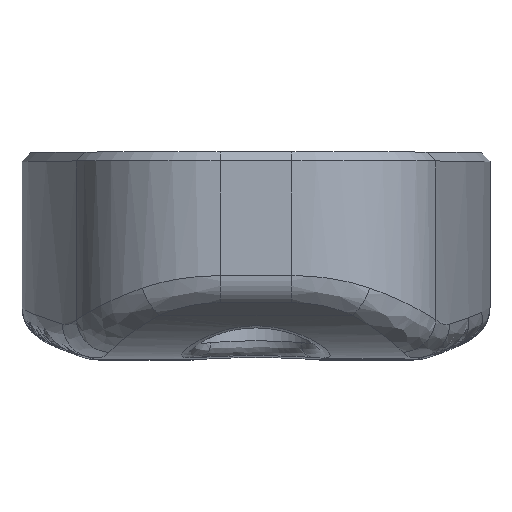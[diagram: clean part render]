
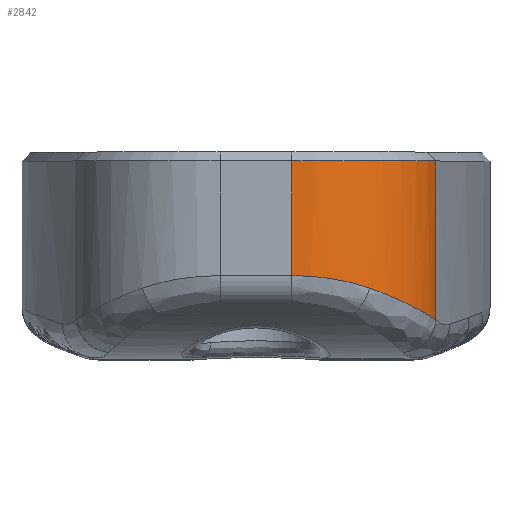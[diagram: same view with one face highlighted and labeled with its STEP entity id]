
A CAD part, top view. The second image highlights one B-rep face of the part: STEP entity #2842.
In plain terms, the highlighted cylindrical face has radius 10 mm (diameter 20 mm), a partial arc.
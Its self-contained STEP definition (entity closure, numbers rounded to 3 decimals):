
#208=LINE('',#6161,#362);
#209=LINE('',#6168,#363);
#362=VECTOR('',#3895,115.186);
#363=VECTOR('',#3898,10.);
#445=CYLINDRICAL_SURFACE('',#3165,10.);
#491=ELLIPSE('',#3166,11.484,10.);
#642=FACE_OUTER_BOUND('',#828,.T.);
#828=EDGE_LOOP('',(#2473,#2474,#2475,#2476,#2477));
#953=B_SPLINE_CURVE_WITH_KNOTS('',3,(#6171,#6172,#6173,#6174,#6175),
 .UNSPECIFIED.,.F.,.F.,(4,1,4),(0.,0.271,0.631),
 .UNSPECIFIED.);
#1103=CIRCLE('',#3154,10.);
#1340=VERTEX_POINT('',#6127);
#1342=VERTEX_POINT('',#6135);
#1347=VERTEX_POINT('',#6160);
#1348=VERTEX_POINT('',#6167);
#1349=VERTEX_POINT('',#6169);
#1726=EDGE_CURVE('',#1340,#1342,#1103,.T.);
#1738=EDGE_CURVE('',#1342,#1347,#208,.T.);
#1740=EDGE_CURVE('',#1340,#1348,#209,.T.);
#1741=EDGE_CURVE('',#1349,#1348,#491,.T.);
#1742=EDGE_CURVE('',#1347,#1349,#953,.T.);
#2473=ORIENTED_EDGE('',*,*,#1726,.F.);
#2474=ORIENTED_EDGE('',*,*,#1740,.T.);
#2475=ORIENTED_EDGE('',*,*,#1741,.F.);
#2476=ORIENTED_EDGE('',*,*,#1742,.F.);
#2477=ORIENTED_EDGE('',*,*,#1738,.F.);
#2842=ADVANCED_FACE('',(#642),#445,.T.);
#3154=AXIS2_PLACEMENT_3D('',#6137,#3865,#3866);
#3165=AXIS2_PLACEMENT_3D('',#6166,#3896,#3897);
#3166=AXIS2_PLACEMENT_3D('',#6170,#3899,#3900);
#3865=DIRECTION('center_axis',(0.,1.,0.));
#3866=DIRECTION('ref_axis',(0.612,0.,0.791));
#3895=DIRECTION('',(0.,-1.,0.));
#3896=DIRECTION('center_axis',(0.,-1.,0.));
#3897=DIRECTION('ref_axis',(0.612,0.,0.791));
#3898=DIRECTION('',(0.,-1.,0.));
#3899=DIRECTION('center_axis',(0.,-0.871,0.492));
#3900=DIRECTION('ref_axis',(0.,0.492,0.871));
#6127=CARTESIAN_POINT('',(102.413,-704.6,132.609));
#6135=CARTESIAN_POINT('',(112.096,-704.6,125.108));
#6137=CARTESIAN_POINT('Origin',(102.413,-704.6,122.609));
#6160=CARTESIAN_POINT('',(112.096,-715.291,125.108));
#6161=CARTESIAN_POINT('',(112.096,-704.,125.108));
#6166=CARTESIAN_POINT('Origin',(102.413,-704.,122.609));
#6167=CARTESIAN_POINT('',(102.413,-712.33,132.609));
#6168=CARTESIAN_POINT('',(102.413,-704.,132.609));
#6169=CARTESIAN_POINT('',(107.657,-713.168,131.124));
#6170=CARTESIAN_POINT('Origin',(102.413,-717.975,122.609));
#6171=CARTESIAN_POINT('Ctrl Pts',(112.096,-715.291,125.108));
#6172=CARTESIAN_POINT('Ctrl Pts',(111.812,-715.096,126.209));
#6173=CARTESIAN_POINT('Ctrl Pts',(110.723,-714.452,128.599));
#6174=CARTESIAN_POINT('Ctrl Pts',(108.891,-713.597,130.364));
#6175=CARTESIAN_POINT('Ctrl Pts',(107.657,-713.168,131.124));
